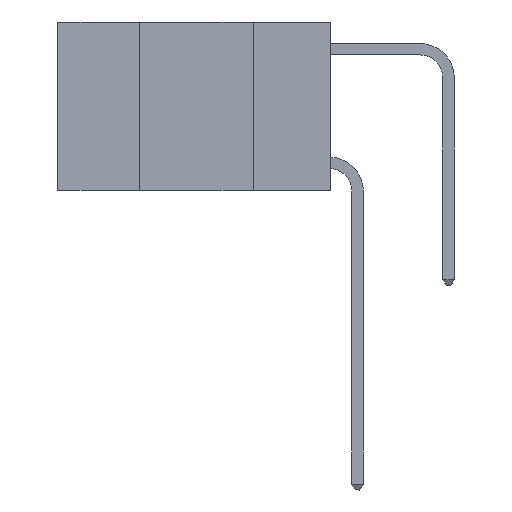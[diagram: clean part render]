
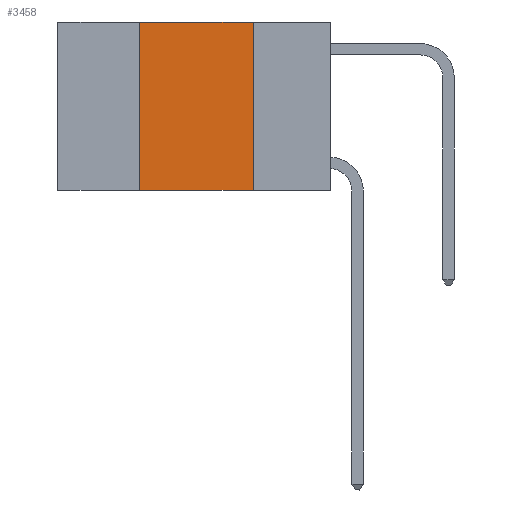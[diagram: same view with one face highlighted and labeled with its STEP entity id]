
A CAD part, left-side view. The second image highlights one B-rep face of the part: STEP entity #3458.
In plain terms, the highlighted planar face has unit normal (-1, 0, 0).
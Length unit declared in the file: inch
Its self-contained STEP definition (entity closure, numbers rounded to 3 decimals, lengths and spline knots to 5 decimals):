
#344 = ORIENTED_EDGE ( 'NONE', *, *, #10584, .F. ) ;
#934 = VERTEX_POINT ( 'NONE', #10886 ) ;
#2064 = EDGE_CURVE ( 'NONE', #11004, #7209, #12934, .T. ) ;
#3458 = ADVANCED_FACE ( 'NONE', ( #6960 ), #10688, .F. ) ;
#5325 = CARTESIAN_POINT ( 'NONE',  ( 0., 0.6, 0. ) ) ;
#6316 = AXIS2_PLACEMENT_3D ( 'NONE', #17486, #19606, #21186 ) ;
#6753 = VERTEX_POINT ( 'NONE', #22227 ) ;
#6950 = CARTESIAN_POINT ( 'NONE',  ( 0., 0.17, 0. ) ) ;
#6960 = FACE_OUTER_BOUND ( 'NONE', #10894, .T. ) ;
#7059 = CARTESIAN_POINT ( 'NONE',  ( 0., 0.42, -0.37 ) ) ;
#7209 = VERTEX_POINT ( 'NONE', #21040 ) ;
#7404 = DIRECTION ( 'NONE',  ( 0., -1., 0. ) ) ;
#8507 = DIRECTION ( 'NONE',  ( 0., 0., -1. ) ) ;
#10584 = EDGE_CURVE ( 'NONE', #7209, #934, #20809, .T. ) ;
#10688 = PLANE ( 'NONE',  #6316 ) ;
#10886 = CARTESIAN_POINT ( 'NONE',  ( 0., 0.17, 0. ) ) ;
#10894 = EDGE_LOOP ( 'NONE', ( #17755, #344, #13124, #19012 ) ) ;
#11004 = VERTEX_POINT ( 'NONE', #7059 ) ;
#12934 = LINE ( 'NONE', #21834, #15983 ) ;
#13124 = ORIENTED_EDGE ( 'NONE', *, *, #2064, .F. ) ;
#14928 = CARTESIAN_POINT ( 'NONE',  ( 0., 0.6, -0.37 ) ) ;
#14938 = EDGE_CURVE ( 'NONE', #11004, #6753, #19726, .T. ) ;
#14956 = VECTOR ( 'NONE', #16705, 39.37008 ) ;
#15983 = VECTOR ( 'NONE', #16115, 39.37008 ) ;
#16115 = DIRECTION ( 'NONE',  ( 0., 0., 1. ) ) ;
#16705 = DIRECTION ( 'NONE',  ( 0., -1., 0. ) ) ;
#17394 = VECTOR ( 'NONE', #7404, 39.37008 ) ;
#17486 = CARTESIAN_POINT ( 'NONE',  ( 0., 0.6, 0. ) ) ;
#17755 = ORIENTED_EDGE ( 'NONE', *, *, #21604, .F. ) ;
#19012 = ORIENTED_EDGE ( 'NONE', *, *, #14938, .T. ) ;
#19606 = DIRECTION ( 'NONE',  ( 1., 0., 0. ) ) ;
#19726 = LINE ( 'NONE', #14928, #14956 ) ;
#20809 = LINE ( 'NONE', #5325, #17394 ) ;
#21040 = CARTESIAN_POINT ( 'NONE',  ( 0., 0.42, 0. ) ) ;
#21186 = DIRECTION ( 'NONE',  ( 0., 0., -1. ) ) ;
#21604 = EDGE_CURVE ( 'NONE', #934, #6753, #22640, .T. ) ;
#21834 = CARTESIAN_POINT ( 'NONE',  ( 0., 0.42, 0. ) ) ;
#22068 = VECTOR ( 'NONE', #8507, 39.37008 ) ;
#22227 = CARTESIAN_POINT ( 'NONE',  ( 0., 0.17, -0.37 ) ) ;
#22640 = LINE ( 'NONE', #6950, #22068 ) ;
